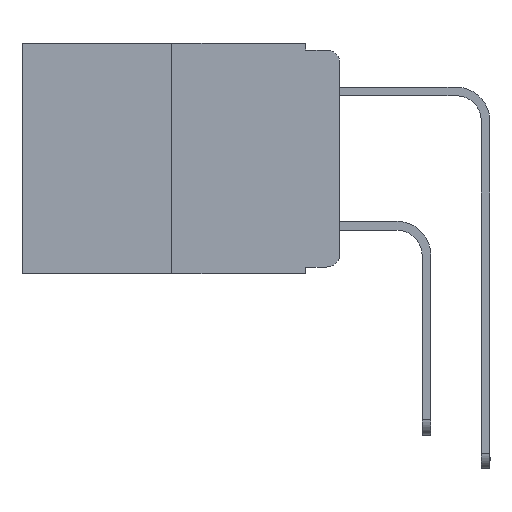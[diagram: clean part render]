
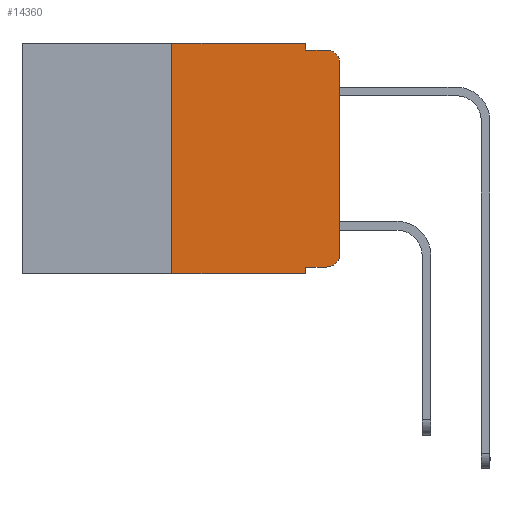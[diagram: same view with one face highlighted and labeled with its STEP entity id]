
A CAD part, left-side view. The second image highlights one B-rep face of the part: STEP entity #14360.
In plain terms, the highlighted planar face has unit normal (-1, 0, 0).
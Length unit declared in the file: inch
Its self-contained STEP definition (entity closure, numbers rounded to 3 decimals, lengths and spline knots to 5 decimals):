
#36 = DIRECTION ( 'NONE',  ( -1., 0., 0. ) ) ;
#247 = VERTEX_POINT ( 'NONE', #14129 ) ;
#514 = ORIENTED_EDGE ( 'NONE', *, *, #3990, .F. ) ;
#729 = LINE ( 'NONE', #16264, #7259 ) ;
#787 = CARTESIAN_POINT ( 'NONE',  ( 0., 0., 0. ) ) ;
#910 = ORIENTED_EDGE ( 'NONE', *, *, #1426, .F. ) ;
#916 = DIRECTION ( 'NONE',  ( 0., -1., 0. ) ) ;
#918 = VERTEX_POINT ( 'NONE', #4434 ) ;
#919 = AXIS2_PLACEMENT_3D ( 'NONE', #7931, #36, #5163 ) ;
#1298 = VERTEX_POINT ( 'NONE', #10566 ) ;
#1426 = EDGE_CURVE ( 'NONE', #13992, #1468, #3143, .T. ) ;
#1468 = VERTEX_POINT ( 'NONE', #13564 ) ;
#1489 = VERTEX_POINT ( 'NONE', #3226 ) ;
#1901 = DIRECTION ( 'NONE',  ( 0., 0., -1. ) ) ;
#1992 = VECTOR ( 'NONE', #10375, 39.37008 ) ;
#2083 = CARTESIAN_POINT ( 'NONE',  ( 0., 0.02, -0.313 ) ) ;
#2254 = DIRECTION ( 'NONE',  ( 0., 0., -1. ) ) ;
#2633 = DIRECTION ( 'NONE',  ( 0., -1., 0. ) ) ;
#2689 = ORIENTED_EDGE ( 'NONE', *, *, #3697, .F. ) ;
#2737 = VERTEX_POINT ( 'NONE', #3565 ) ;
#2920 = EDGE_CURVE ( 'NONE', #3374, #247, #5174, .T. ) ;
#2975 = VECTOR ( 'NONE', #916, 39.37008 ) ;
#3143 = LINE ( 'NONE', #13387, #3210 ) ;
#3210 = VECTOR ( 'NONE', #1901, 39.37008 ) ;
#3226 = CARTESIAN_POINT ( 'NONE',  ( 0., 0., -0.03 ) ) ;
#3374 = VERTEX_POINT ( 'NONE', #4402 ) ;
#3376 = LINE ( 'NONE', #787, #11084 ) ;
#3543 = DIRECTION ( 'NONE',  ( 0., 0., 1. ) ) ;
#3565 = CARTESIAN_POINT ( 'NONE',  ( 0., 0.051, -0.343 ) ) ;
#3697 = EDGE_CURVE ( 'NONE', #247, #13992, #9073, .T. ) ;
#3766 = DIRECTION ( 'NONE',  ( 1., 0., 0. ) ) ;
#3990 = EDGE_CURVE ( 'NONE', #8503, #2737, #5892, .T. ) ;
#4249 = VERTEX_POINT ( 'NONE', #13267 ) ;
#4402 = CARTESIAN_POINT ( 'NONE',  ( 0., 0.25, -0.343 ) ) ;
#4434 = CARTESIAN_POINT ( 'NONE',  ( 0., 0., -0.313 ) ) ;
#4744 = DIRECTION ( 'NONE',  ( 0., -1., 0. ) ) ;
#4753 = CARTESIAN_POINT ( 'NONE',  ( 0., 0.473, -0.343 ) ) ;
#4990 = ORIENTED_EDGE ( 'NONE', *, *, #12317, .T. ) ;
#5057 = ORIENTED_EDGE ( 'NONE', *, *, #2920, .F. ) ;
#5129 = PLANE ( 'NONE',  #9148 ) ;
#5163 = DIRECTION ( 'NONE',  ( 0., 0., -1. ) ) ;
#5174 = LINE ( 'NONE', #8843, #1992 ) ;
#5892 = LINE ( 'NONE', #16379, #14747 ) ;
#7215 = ORIENTED_EDGE ( 'NONE', *, *, #12094, .T. ) ;
#7259 = VECTOR ( 'NONE', #4744, 39.37008 ) ;
#7741 = DIRECTION ( 'NONE',  ( 0., -1., 0. ) ) ;
#7931 = CARTESIAN_POINT ( 'NONE',  ( 0., 0.02, -0.03 ) ) ;
#8298 = EDGE_CURVE ( 'NONE', #1489, #1298, #12731, .T. ) ;
#8411 = DIRECTION ( 'NONE',  ( 0., 0., -1. ) ) ;
#8503 = VERTEX_POINT ( 'NONE', #14820 ) ;
#8832 = ORIENTED_EDGE ( 'NONE', *, *, #10684, .T. ) ;
#8843 = CARTESIAN_POINT ( 'NONE',  ( 0., 0.25, 0. ) ) ;
#9073 = LINE ( 'NONE', #11453, #9156 ) ;
#9148 = AXIS2_PLACEMENT_3D ( 'NONE', #15292, #3766, #10257 ) ;
#9156 = VECTOR ( 'NONE', #7741, 39.37008 ) ;
#9398 = EDGE_CURVE ( 'NONE', #4249, #918, #11378, .T. ) ;
#10163 = FACE_OUTER_BOUND ( 'NONE', #10211, .T. ) ;
#10211 = EDGE_LOOP ( 'NONE', ( #4990, #11300, #16254, #910, #2689, #5057, #8832, #514, #7215, #10659 ) ) ;
#10257 = DIRECTION ( 'NONE',  ( 0., 0., -1. ) ) ;
#10375 = DIRECTION ( 'NONE',  ( 0., 0., 1. ) ) ;
#10566 = CARTESIAN_POINT ( 'NONE',  ( 0., 0.02, -0.01 ) ) ;
#10659 = ORIENTED_EDGE ( 'NONE', *, *, #9398, .T. ) ;
#10684 = EDGE_CURVE ( 'NONE', #3374, #2737, #16108, .T. ) ;
#11084 = VECTOR ( 'NONE', #3543, 39.37008 ) ;
#11300 = ORIENTED_EDGE ( 'NONE', *, *, #8298, .T. ) ;
#11378 = CIRCLE ( 'NONE', #13236, 0.02 ) ;
#11453 = CARTESIAN_POINT ( 'NONE',  ( 0., 0.473, 0. ) ) ;
#11887 = VECTOR ( 'NONE', #2633, 39.37008 ) ;
#12094 = EDGE_CURVE ( 'NONE', #8503, #4249, #15503, .T. ) ;
#12317 = EDGE_CURVE ( 'NONE', #918, #1489, #3376, .T. ) ;
#12731 = CIRCLE ( 'NONE', #919, 0.02 ) ;
#12740 = CARTESIAN_POINT ( 'NONE',  ( 0., 0.051, -0.333 ) ) ;
#13236 = AXIS2_PLACEMENT_3D ( 'NONE', #2083, #14935, #2254 ) ;
#13267 = CARTESIAN_POINT ( 'NONE',  ( 0., 0.02, -0.333 ) ) ;
#13387 = CARTESIAN_POINT ( 'NONE',  ( 0., 0.051, 0. ) ) ;
#13564 = CARTESIAN_POINT ( 'NONE',  ( 0., 0.051, -0.01 ) ) ;
#13797 = EDGE_CURVE ( 'NONE', #1468, #1298, #729, .T. ) ;
#13992 = VERTEX_POINT ( 'NONE', #15904 ) ;
#14129 = CARTESIAN_POINT ( 'NONE',  ( 0., 0.25, 0. ) ) ;
#14360 = ADVANCED_FACE ( 'NONE', ( #10163 ), #5129, .F. ) ;
#14747 = VECTOR ( 'NONE', #8411, 39.37008 ) ;
#14820 = CARTESIAN_POINT ( 'NONE',  ( 0., 0.051, -0.333 ) ) ;
#14935 = DIRECTION ( 'NONE',  ( -1., 0., 0. ) ) ;
#15292 = CARTESIAN_POINT ( 'NONE',  ( 0., 0.473, 0. ) ) ;
#15503 = LINE ( 'NONE', #12740, #11887 ) ;
#15904 = CARTESIAN_POINT ( 'NONE',  ( 0., 0.051, 0. ) ) ;
#16108 = LINE ( 'NONE', #4753, #2975 ) ;
#16254 = ORIENTED_EDGE ( 'NONE', *, *, #13797, .F. ) ;
#16264 = CARTESIAN_POINT ( 'NONE',  ( 0., 0.051, -0.01 ) ) ;
#16379 = CARTESIAN_POINT ( 'NONE',  ( 0., 0.051, 0. ) ) ;
